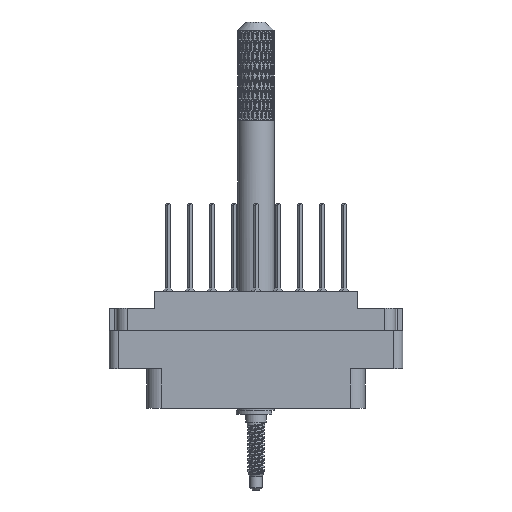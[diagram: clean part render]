
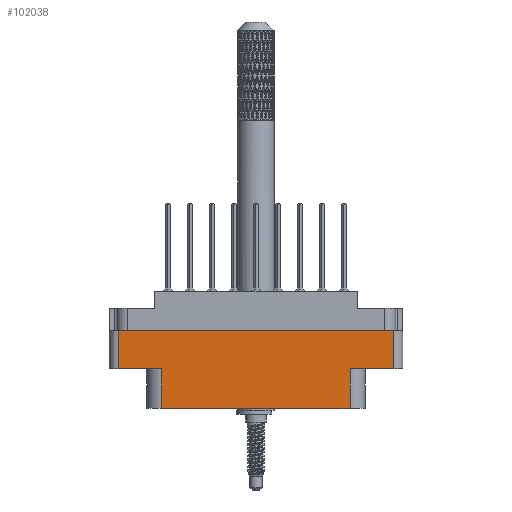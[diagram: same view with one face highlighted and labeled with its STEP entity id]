
A CAD part, front view. The second image highlights one B-rep face of the part: STEP entity #102038.
In plain terms, the highlighted planar face has unit normal (0, -1, 0).
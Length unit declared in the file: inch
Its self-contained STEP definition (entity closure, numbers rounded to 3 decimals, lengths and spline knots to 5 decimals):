
#426 = AXIS2_PLACEMENT_3D ( 'NONE', #42664, #66415, #73751 ) ;
#2134 = CARTESIAN_POINT ( 'NONE',  ( -0.938, -0.438, -0.798 ) ) ;
#2165 = EDGE_CURVE ( 'NONE', #21383, #33995, #12508, .T. ) ;
#4213 = ORIENTED_EDGE ( 'NONE', *, *, #73913, .F. ) ;
#4451 = DIRECTION ( 'NONE',  ( 0., 0., 1. ) ) ;
#7437 = VECTOR ( 'NONE', #58418, 39.37008 ) ;
#10421 = VECTOR ( 'NONE', #18734, 39.37008 ) ;
#11054 = VERTEX_POINT ( 'NONE', #92300 ) ;
#12439 = ORIENTED_EDGE ( 'NONE', *, *, #39138, .F. ) ;
#12508 = LINE ( 'NONE', #35582, #49510 ) ;
#13368 = LINE ( 'NONE', #47063, #68958 ) ;
#13402 = LINE ( 'NONE', #58865, #29481 ) ;
#14004 = VECTOR ( 'NONE', #82259, 39.37008 ) ;
#15086 = CARTESIAN_POINT ( 'NONE',  ( 0.938, -0.438, -0.268 ) ) ;
#16208 = CARTESIAN_POINT ( 'NONE',  ( 0.938, -0.438, -0.529 ) ) ;
#18734 = DIRECTION ( 'NONE',  ( 0., 0., -1. ) ) ;
#19479 = CARTESIAN_POINT ( 'NONE',  ( -0.938, -0.438, -0.268 ) ) ;
#19490 = PLANE ( 'NONE',  #426 ) ;
#21383 = VERTEX_POINT ( 'NONE', #16208 ) ;
#23593 = VERTEX_POINT ( 'NONE', #56397 ) ;
#25295 = LINE ( 'NONE', #27371, #10421 ) ;
#25442 = CARTESIAN_POINT ( 'NONE',  ( 0.644, -0.438, -0.798 ) ) ;
#26624 = DIRECTION ( 'NONE',  ( 1., 0., 0. ) ) ;
#26994 = CARTESIAN_POINT ( 'NONE',  ( -1., -0.438, -0.268 ) ) ;
#27371 = CARTESIAN_POINT ( 'NONE',  ( -0.644, -0.438, -0.529 ) ) ;
#29013 = EDGE_CURVE ( 'NONE', #11054, #93382, #25295, .T. ) ;
#29481 = VECTOR ( 'NONE', #34083, 39.37008 ) ;
#33995 = VERTEX_POINT ( 'NONE', #15086 ) ;
#34083 = DIRECTION ( 'NONE',  ( 0., 0., 1. ) ) ;
#35582 = CARTESIAN_POINT ( 'NONE',  ( 0.938, -0.438, -0.798 ) ) ;
#36193 = VERTEX_POINT ( 'NONE', #19479 ) ;
#38665 = EDGE_LOOP ( 'NONE', ( #49602, #89519, #4213, #79346, #50545, #12439, #44739, #85099 ) ) ;
#39138 = EDGE_CURVE ( 'NONE', #36193, #33995, #54838, .T. ) ;
#42664 = CARTESIAN_POINT ( 'NONE',  ( -0.938, -0.438, -0.798 ) ) ;
#44739 = ORIENTED_EDGE ( 'NONE', *, *, #89433, .F. ) ;
#45382 = DIRECTION ( 'NONE',  ( 0., 0., -1. ) ) ;
#47063 = CARTESIAN_POINT ( 'NONE',  ( 0., -0.438, -0.529 ) ) ;
#49510 = VECTOR ( 'NONE', #4451, 39.37008 ) ;
#49602 = ORIENTED_EDGE ( 'NONE', *, *, #29013, .T. ) ;
#50545 = ORIENTED_EDGE ( 'NONE', *, *, #2165, .T. ) ;
#51638 = CARTESIAN_POINT ( 'NONE',  ( 0.644, -0.438, -0.529 ) ) ;
#52776 = VECTOR ( 'NONE', #45382, 39.37008 ) ;
#53897 = EDGE_CURVE ( 'NONE', #97571, #11054, #80362, .T. ) ;
#54838 = LINE ( 'NONE', #26994, #14004 ) ;
#56397 = CARTESIAN_POINT ( 'NONE',  ( 0.644, -0.438, -0.529 ) ) ;
#58086 = CARTESIAN_POINT ( 'NONE',  ( 0., -0.438, -0.529 ) ) ;
#58418 = DIRECTION ( 'NONE',  ( 1., 0., 0. ) ) ;
#58713 = FACE_OUTER_BOUND ( 'NONE', #38665, .T. ) ;
#58865 = CARTESIAN_POINT ( 'NONE',  ( -0.938, -0.438, -0.798 ) ) ;
#60605 = CARTESIAN_POINT ( 'NONE',  ( -0.938, -0.438, -0.529 ) ) ;
#66415 = DIRECTION ( 'NONE',  ( 0., -1., 0. ) ) ;
#68958 = VECTOR ( 'NONE', #102305, 39.37008 ) ;
#70918 = EDGE_CURVE ( 'NONE', #93382, #73750, #81245, .T. ) ;
#73750 = VERTEX_POINT ( 'NONE', #25442 ) ;
#73751 = DIRECTION ( 'NONE',  ( 0., 0., -1. ) ) ;
#73913 = EDGE_CURVE ( 'NONE', #23593, #73750, #102189, .T. ) ;
#79346 = ORIENTED_EDGE ( 'NONE', *, *, #99634, .F. ) ;
#80362 = LINE ( 'NONE', #58086, #7437 ) ;
#81245 = LINE ( 'NONE', #2134, #98567 ) ;
#82259 = DIRECTION ( 'NONE',  ( 1., 0., 0. ) ) ;
#85099 = ORIENTED_EDGE ( 'NONE', *, *, #53897, .T. ) ;
#89433 = EDGE_CURVE ( 'NONE', #97571, #36193, #13402, .T. ) ;
#89519 = ORIENTED_EDGE ( 'NONE', *, *, #70918, .T. ) ;
#92300 = CARTESIAN_POINT ( 'NONE',  ( -0.644, -0.438, -0.529 ) ) ;
#93382 = VERTEX_POINT ( 'NONE', #100770 ) ;
#97571 = VERTEX_POINT ( 'NONE', #60605 ) ;
#98567 = VECTOR ( 'NONE', #26624, 39.37008 ) ;
#99634 = EDGE_CURVE ( 'NONE', #21383, #23593, #13368, .T. ) ;
#100770 = CARTESIAN_POINT ( 'NONE',  ( -0.644, -0.438, -0.798 ) ) ;
#102038 = ADVANCED_FACE ( 'NONE', ( #58713 ), #19490, .T. ) ;
#102189 = LINE ( 'NONE', #51638, #52776 ) ;
#102305 = DIRECTION ( 'NONE',  ( -1., 0., 0. ) ) ;
